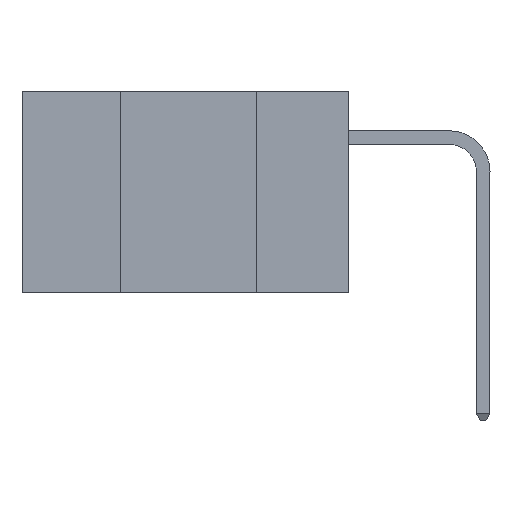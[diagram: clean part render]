
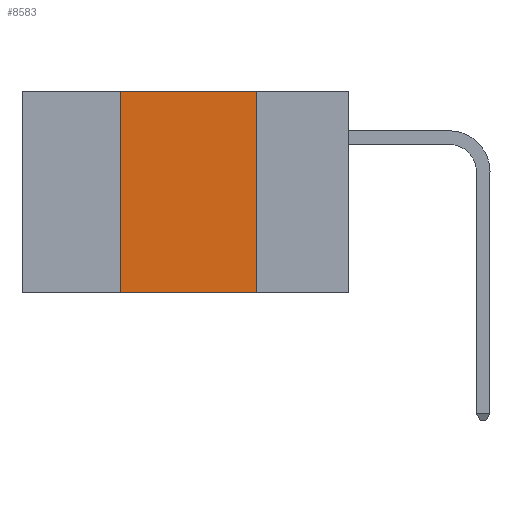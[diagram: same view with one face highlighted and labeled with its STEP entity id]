
A CAD part, left-side view. The second image highlights one B-rep face of the part: STEP entity #8583.
In plain terms, the highlighted planar face has unit normal (-1, 0, 0).
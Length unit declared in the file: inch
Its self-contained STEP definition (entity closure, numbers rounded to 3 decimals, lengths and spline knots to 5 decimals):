
#2305 = LINE ( 'NONE', #32276, #9905 ) ;
#2644 = CARTESIAN_POINT ( 'NONE',  ( 0., 0.42, -0.37 ) ) ;
#3625 = CARTESIAN_POINT ( 'NONE',  ( 0., 0.6, 0. ) ) ;
#3652 = EDGE_CURVE ( 'NONE', #8182, #22289, #30722, .T. ) ;
#5355 = DIRECTION ( 'NONE',  ( 0., -1., 0. ) ) ;
#6471 = DIRECTION ( 'NONE',  ( 1., 0., 0. ) ) ;
#8182 = VERTEX_POINT ( 'NONE', #15981 ) ;
#8583 = ADVANCED_FACE ( 'NONE', ( #33794 ), #9240, .F. ) ;
#9240 = PLANE ( 'NONE',  #21478 ) ;
#9270 = VECTOR ( 'NONE', #32868, 39.37008 ) ;
#9905 = VECTOR ( 'NONE', #35035, 39.37008 ) ;
#12137 = VECTOR ( 'NONE', #5355, 39.37008 ) ;
#12411 = EDGE_CURVE ( 'NONE', #17576, #15506, #20561, .T. ) ;
#13412 = CARTESIAN_POINT ( 'NONE',  ( 0., 0.42, 0. ) ) ;
#14461 = ORIENTED_EDGE ( 'NONE', *, *, #29297, .F. ) ;
#15506 = VERTEX_POINT ( 'NONE', #35223 ) ;
#15705 = CARTESIAN_POINT ( 'NONE',  ( 0., 0.17, 0. ) ) ;
#15981 = CARTESIAN_POINT ( 'NONE',  ( 0., 0.42, 0. ) ) ;
#15990 = VECTOR ( 'NONE', #30147, 39.37008 ) ;
#16076 = ORIENTED_EDGE ( 'NONE', *, *, #3652, .F. ) ;
#16935 = ORIENTED_EDGE ( 'NONE', *, *, #18151, .F. ) ;
#17576 = VERTEX_POINT ( 'NONE', #2644 ) ;
#18151 = EDGE_CURVE ( 'NONE', #17576, #8182, #29910, .T. ) ;
#20561 = LINE ( 'NONE', #35897, #12137 ) ;
#21478 = AXIS2_PLACEMENT_3D ( 'NONE', #3625, #6471, #26152 ) ;
#22289 = VERTEX_POINT ( 'NONE', #15705 ) ;
#23489 = EDGE_LOOP ( 'NONE', ( #14461, #16076, #16935, #25895 ) ) ;
#25895 = ORIENTED_EDGE ( 'NONE', *, *, #12411, .T. ) ;
#26152 = DIRECTION ( 'NONE',  ( 0., 0., -1. ) ) ;
#29297 = EDGE_CURVE ( 'NONE', #22289, #15506, #2305, .T. ) ;
#29910 = LINE ( 'NONE', #13412, #15990 ) ;
#30147 = DIRECTION ( 'NONE',  ( 0., 0., 1. ) ) ;
#30722 = LINE ( 'NONE', #32626, #9270 ) ;
#32276 = CARTESIAN_POINT ( 'NONE',  ( 0., 0.17, 0. ) ) ;
#32626 = CARTESIAN_POINT ( 'NONE',  ( 0., 0.6, 0. ) ) ;
#32868 = DIRECTION ( 'NONE',  ( 0., -1., 0. ) ) ;
#33794 = FACE_OUTER_BOUND ( 'NONE', #23489, .T. ) ;
#35035 = DIRECTION ( 'NONE',  ( 0., 0., -1. ) ) ;
#35223 = CARTESIAN_POINT ( 'NONE',  ( 0., 0.17, -0.37 ) ) ;
#35897 = CARTESIAN_POINT ( 'NONE',  ( 0., 0.6, -0.37 ) ) ;
